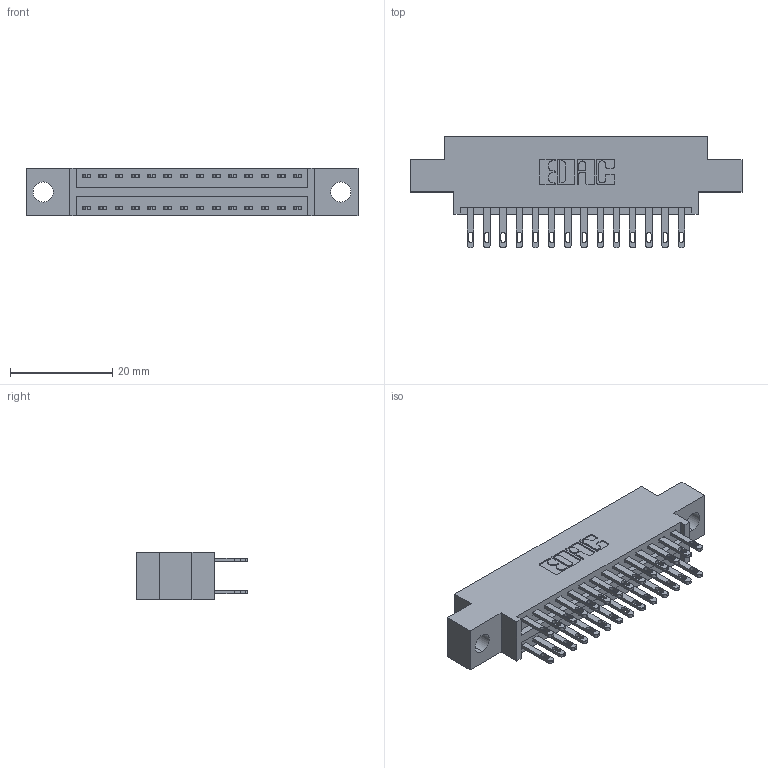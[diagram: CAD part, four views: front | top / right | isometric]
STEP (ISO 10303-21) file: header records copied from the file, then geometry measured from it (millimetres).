
FILE_DESCRIPTION (( 'STEP AP203' ), '1' );
FILE_NAME ('346-028-500-804.STEP', '2022-05-19T03:26:06', ( '' ), ( '' ), 'SwSTEP 2.0', 'SolidWorks 2020', '' );
FILE_SCHEMA (( 'CONFIG_CONTROL_DESIGN' ));
Length unit declared in the file: inch
Products named in the file (3): 345-292-001_345-293-100; 346 Part_0.170 Offset - 0.156 Dia-TH; 346-028-500-804
Assembly tree (29 placements, depth 2):
  346-028-500-804
    346 Part_0.170 Offset - 0.156 Dia-TH
    345-292-001_345-293-100  x28
Bounding box: 65.02 x 21.84 x 9.4 mm (x, y, z)
Volume: 5948.2 mm3; surface area: 8056.7 mm2
Topology: 29 solids, 29 shells, 1484 faces, 4493 edges, 2994 vertices
Faces by surface type: plane 906, cylinder 578
Entity records: 13387 total; most frequent: CARTESIAN_POINT 2250, ORIENTED_EDGE 2182, DIRECTION 2035, EDGE_CURVE 1091, LINE 899, VECTOR 899, VERTEX_POINT 726, AXIS2_PLACEMENT_3D 568
